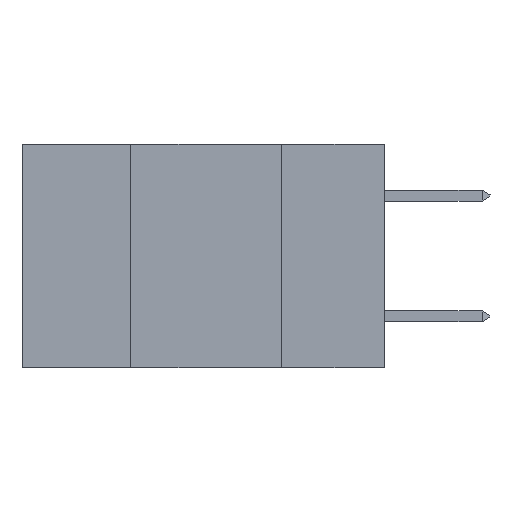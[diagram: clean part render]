
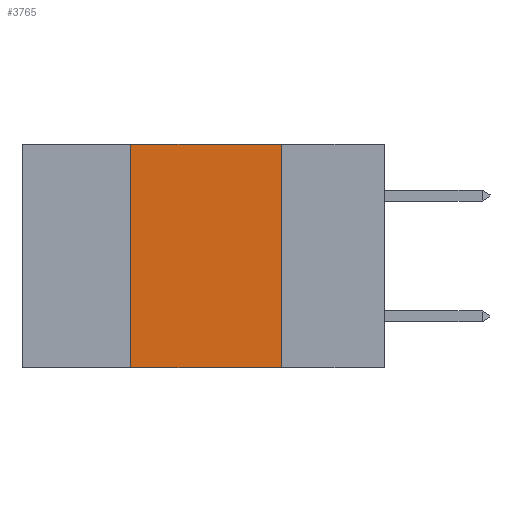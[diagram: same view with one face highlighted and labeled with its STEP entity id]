
A CAD part, left-side view. The second image highlights one B-rep face of the part: STEP entity #3765.
In plain terms, the highlighted planar face has unit normal (-1, 0, 0).
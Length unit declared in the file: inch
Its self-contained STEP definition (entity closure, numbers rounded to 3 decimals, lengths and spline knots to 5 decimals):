
#1626 = CARTESIAN_POINT ( 'NONE',  ( 0., 0.6, 0. ) ) ;
#3765 = ADVANCED_FACE ( 'NONE', ( #25459 ), #37845, .F. ) ;
#3889 = DIRECTION ( 'NONE',  ( 0., 0., -1. ) ) ;
#5598 = EDGE_CURVE ( 'NONE', #36740, #12807, #26441, .T. ) ;
#6015 = ORIENTED_EDGE ( 'NONE', *, *, #12695, .T. ) ;
#6171 = CARTESIAN_POINT ( 'NONE',  ( 0., 0.17, 0. ) ) ;
#6558 = DIRECTION ( 'NONE',  ( 0., -1., 0. ) ) ;
#7737 = LINE ( 'NONE', #32163, #17412 ) ;
#9999 = CARTESIAN_POINT ( 'NONE',  ( 0., 0.6, 0. ) ) ;
#12088 = LINE ( 'NONE', #15141, #12232 ) ;
#12232 = VECTOR ( 'NONE', #36891, 39.37008 ) ;
#12543 = CARTESIAN_POINT ( 'NONE',  ( 0., 0.42, -0.37 ) ) ;
#12695 = EDGE_CURVE ( 'NONE', #26736, #30339, #34205, .T. ) ;
#12807 = VERTEX_POINT ( 'NONE', #6171 ) ;
#14995 = CARTESIAN_POINT ( 'NONE',  ( 0., 0.42, 0. ) ) ;
#15141 = CARTESIAN_POINT ( 'NONE',  ( 0., 0.42, 0. ) ) ;
#17320 = ORIENTED_EDGE ( 'NONE', *, *, #5598, .F. ) ;
#17412 = VECTOR ( 'NONE', #3889, 39.37008 ) ;
#18268 = EDGE_LOOP ( 'NONE', ( #29190, #17320, #30909, #6015 ) ) ;
#19811 = VECTOR ( 'NONE', #6558, 39.37008 ) ;
#22393 = DIRECTION ( 'NONE',  ( 1., 0., 0. ) ) ;
#25432 = VECTOR ( 'NONE', #39226, 39.37008 ) ;
#25459 = FACE_OUTER_BOUND ( 'NONE', #18268, .T. ) ;
#25999 = CARTESIAN_POINT ( 'NONE',  ( 0., 0.17, -0.37 ) ) ;
#26441 = LINE ( 'NONE', #1626, #25432 ) ;
#26736 = VERTEX_POINT ( 'NONE', #12543 ) ;
#28535 = EDGE_CURVE ( 'NONE', #26736, #36740, #12088, .T. ) ;
#29190 = ORIENTED_EDGE ( 'NONE', *, *, #34703, .F. ) ;
#30339 = VERTEX_POINT ( 'NONE', #25999 ) ;
#30909 = ORIENTED_EDGE ( 'NONE', *, *, #28535, .F. ) ;
#30970 = CARTESIAN_POINT ( 'NONE',  ( 0., 0.6, -0.37 ) ) ;
#32163 = CARTESIAN_POINT ( 'NONE',  ( 0., 0.17, 0. ) ) ;
#34205 = LINE ( 'NONE', #30970, #19811 ) ;
#34703 = EDGE_CURVE ( 'NONE', #12807, #30339, #7737, .T. ) ;
#34803 = DIRECTION ( 'NONE',  ( 0., 0., -1. ) ) ;
#35700 = AXIS2_PLACEMENT_3D ( 'NONE', #9999, #22393, #34803 ) ;
#36740 = VERTEX_POINT ( 'NONE', #14995 ) ;
#36891 = DIRECTION ( 'NONE',  ( 0., 0., 1. ) ) ;
#37845 = PLANE ( 'NONE',  #35700 ) ;
#39226 = DIRECTION ( 'NONE',  ( 0., -1., 0. ) ) ;
